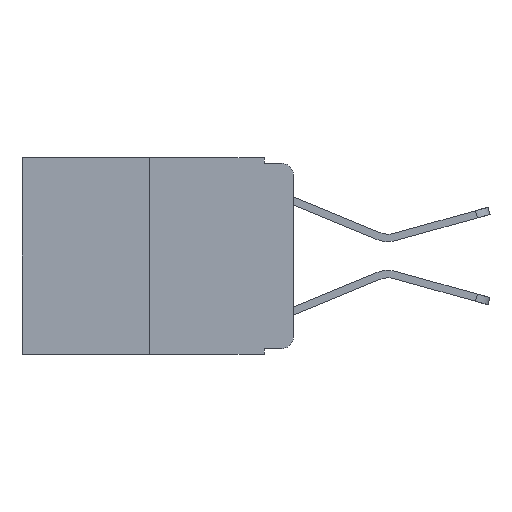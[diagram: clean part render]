
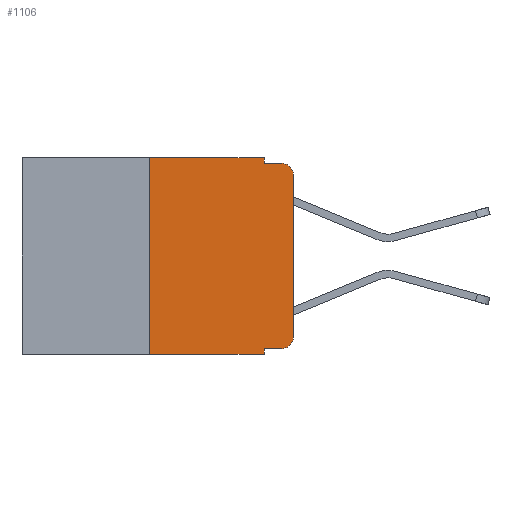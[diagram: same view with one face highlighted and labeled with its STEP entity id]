
A CAD part, left-side view. The second image highlights one B-rep face of the part: STEP entity #1106.
In plain terms, the highlighted planar face has unit normal (-1, 0, 0).
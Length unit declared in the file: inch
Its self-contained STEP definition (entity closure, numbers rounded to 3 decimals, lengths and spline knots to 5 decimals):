
#6 = EDGE_LOOP ( 'NONE', ( #10624, #8371, #10915, #5962, #11212, #8969, #1506, #9570, #4493, #10180 ) ) ;
#286 = DIRECTION ( 'NONE',  ( 0., 0., -1. ) ) ;
#703 = VERTEX_POINT ( 'NONE', #9747 ) ;
#732 = CIRCLE ( 'NONE', #8877, 0.02 ) ;
#757 = CARTESIAN_POINT ( 'NONE',  ( 0., 0.051, 0. ) ) ;
#875 = VECTOR ( 'NONE', #8287, 39.37008 ) ;
#1106 = ADVANCED_FACE ( 'NONE', ( #9451 ), #7202, .F. ) ;
#1124 = VERTEX_POINT ( 'NONE', #11793 ) ;
#1135 = CARTESIAN_POINT ( 'NONE',  ( 0., 0.25, 0. ) ) ;
#1459 = CARTESIAN_POINT ( 'NONE',  ( 0., 0.051, -0.333 ) ) ;
#1506 = ORIENTED_EDGE ( 'NONE', *, *, #10758, .T. ) ;
#1712 = VECTOR ( 'NONE', #12233, 39.37008 ) ;
#1839 = EDGE_CURVE ( 'NONE', #8189, #5122, #732, .T. ) ;
#1941 = VERTEX_POINT ( 'NONE', #3973 ) ;
#2005 = DIRECTION ( 'NONE',  ( 0., 0., -1. ) ) ;
#2023 = LINE ( 'NONE', #11300, #1712 ) ;
#2132 = DIRECTION ( 'NONE',  ( 0., 0., 1. ) ) ;
#2383 = CARTESIAN_POINT ( 'NONE',  ( 0., 0.02, -0.313 ) ) ;
#2522 = EDGE_CURVE ( 'NONE', #4773, #8189, #6657, .T. ) ;
#2772 = CARTESIAN_POINT ( 'NONE',  ( 0., 0.02, -0.01 ) ) ;
#2823 = CARTESIAN_POINT ( 'NONE',  ( 0., 0.25, -0.343 ) ) ;
#2832 = EDGE_CURVE ( 'NONE', #12515, #1941, #11077, .T. ) ;
#2888 = DIRECTION ( 'NONE',  ( -1., 0., 0. ) ) ;
#3226 = AXIS2_PLACEMENT_3D ( 'NONE', #11378, #6931, #4827 ) ;
#3488 = CARTESIAN_POINT ( 'NONE',  ( 0., 0., 0. ) ) ;
#3854 = EDGE_CURVE ( 'NONE', #4773, #4726, #10399, .T. ) ;
#3973 = CARTESIAN_POINT ( 'NONE',  ( 0., 0.051, 0. ) ) ;
#4180 = CARTESIAN_POINT ( 'NONE',  ( 0., 0.473, 0. ) ) ;
#4339 = VECTOR ( 'NONE', #4501, 39.37008 ) ;
#4493 = ORIENTED_EDGE ( 'NONE', *, *, #2522, .T. ) ;
#4501 = DIRECTION ( 'NONE',  ( 0., 0., 1. ) ) ;
#4542 = EDGE_CURVE ( 'NONE', #5656, #12515, #8275, .T. ) ;
#4726 = VERTEX_POINT ( 'NONE', #11400 ) ;
#4769 = LINE ( 'NONE', #8827, #9831 ) ;
#4773 = VERTEX_POINT ( 'NONE', #10484 ) ;
#4827 = DIRECTION ( 'NONE',  ( 0., 0., -1. ) ) ;
#5122 = VERTEX_POINT ( 'NONE', #8151 ) ;
#5226 = EDGE_CURVE ( 'NONE', #1941, #1124, #10670, .T. ) ;
#5342 = VECTOR ( 'NONE', #8292, 39.37008 ) ;
#5656 = VERTEX_POINT ( 'NONE', #2823 ) ;
#5799 = CARTESIAN_POINT ( 'NONE',  ( 0., 0.25, 0. ) ) ;
#5854 = AXIS2_PLACEMENT_3D ( 'NONE', #12269, #6437, #286 ) ;
#5880 = DIRECTION ( 'NONE',  ( 0., 0., -1. ) ) ;
#5962 = ORIENTED_EDGE ( 'NONE', *, *, #5226, .F. ) ;
#6437 = DIRECTION ( 'NONE',  ( -1., 0., 0. ) ) ;
#6657 = LINE ( 'NONE', #1459, #875 ) ;
#6931 = DIRECTION ( 'NONE',  ( 1., 0., 0. ) ) ;
#7091 = LINE ( 'NONE', #3488, #4339 ) ;
#7202 = PLANE ( 'NONE',  #3226 ) ;
#7943 = VECTOR ( 'NONE', #2132, 39.37008 ) ;
#7994 = EDGE_CURVE ( 'NONE', #1124, #10809, #2023, .T. ) ;
#8151 = CARTESIAN_POINT ( 'NONE',  ( 0., 0., -0.313 ) ) ;
#8189 = VERTEX_POINT ( 'NONE', #12493 ) ;
#8275 = LINE ( 'NONE', #1135, #7943 ) ;
#8287 = DIRECTION ( 'NONE',  ( 0., -1., 0. ) ) ;
#8292 = DIRECTION ( 'NONE',  ( 0., 0., -1. ) ) ;
#8371 = ORIENTED_EDGE ( 'NONE', *, *, #8668, .T. ) ;
#8529 = VECTOR ( 'NONE', #11176, 39.37008 ) ;
#8668 = EDGE_CURVE ( 'NONE', #703, #10809, #9893, .T. ) ;
#8827 = CARTESIAN_POINT ( 'NONE',  ( 0., 0.473, -0.343 ) ) ;
#8877 = AXIS2_PLACEMENT_3D ( 'NONE', #2383, #2888, #2005 ) ;
#8969 = ORIENTED_EDGE ( 'NONE', *, *, #4542, .F. ) ;
#9316 = EDGE_CURVE ( 'NONE', #5122, #703, #7091, .T. ) ;
#9451 = FACE_OUTER_BOUND ( 'NONE', #6, .T. ) ;
#9570 = ORIENTED_EDGE ( 'NONE', *, *, #3854, .F. ) ;
#9747 = CARTESIAN_POINT ( 'NONE',  ( 0., 0., -0.03 ) ) ;
#9802 = DIRECTION ( 'NONE',  ( 0., -1., 0. ) ) ;
#9831 = VECTOR ( 'NONE', #9802, 39.37008 ) ;
#9893 = CIRCLE ( 'NONE', #5854, 0.02 ) ;
#10180 = ORIENTED_EDGE ( 'NONE', *, *, #1839, .T. ) ;
#10399 = LINE ( 'NONE', #757, #12623 ) ;
#10484 = CARTESIAN_POINT ( 'NONE',  ( 0., 0.051, -0.333 ) ) ;
#10624 = ORIENTED_EDGE ( 'NONE', *, *, #9316, .T. ) ;
#10670 = LINE ( 'NONE', #11177, #5342 ) ;
#10758 = EDGE_CURVE ( 'NONE', #5656, #4726, #4769, .T. ) ;
#10809 = VERTEX_POINT ( 'NONE', #2772 ) ;
#10915 = ORIENTED_EDGE ( 'NONE', *, *, #7994, .F. ) ;
#11077 = LINE ( 'NONE', #4180, #8529 ) ;
#11176 = DIRECTION ( 'NONE',  ( 0., -1., 0. ) ) ;
#11177 = CARTESIAN_POINT ( 'NONE',  ( 0., 0.051, 0. ) ) ;
#11212 = ORIENTED_EDGE ( 'NONE', *, *, #2832, .F. ) ;
#11300 = CARTESIAN_POINT ( 'NONE',  ( 0., 0.051, -0.01 ) ) ;
#11378 = CARTESIAN_POINT ( 'NONE',  ( 0., 0.473, 0. ) ) ;
#11400 = CARTESIAN_POINT ( 'NONE',  ( 0., 0.051, -0.343 ) ) ;
#11793 = CARTESIAN_POINT ( 'NONE',  ( 0., 0.051, -0.01 ) ) ;
#12233 = DIRECTION ( 'NONE',  ( 0., -1., 0. ) ) ;
#12269 = CARTESIAN_POINT ( 'NONE',  ( 0., 0.02, -0.03 ) ) ;
#12493 = CARTESIAN_POINT ( 'NONE',  ( 0., 0.02, -0.333 ) ) ;
#12515 = VERTEX_POINT ( 'NONE', #5799 ) ;
#12623 = VECTOR ( 'NONE', #5880, 39.37008 ) ;
